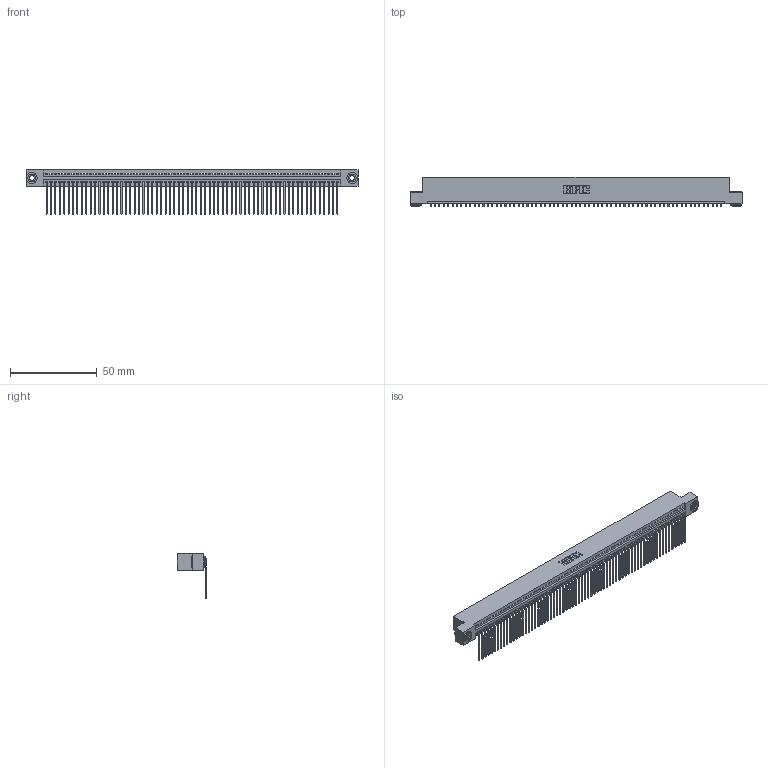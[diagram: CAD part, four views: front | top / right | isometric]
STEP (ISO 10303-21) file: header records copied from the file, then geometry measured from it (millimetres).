
FILE_DESCRIPTION (( 'STEP AP203' ), '1' );
FILE_NAME ('345-067-559-103.STEP', '2018-09-29T05:28:44', ( '' ), ( '' ), 'SwSTEP 2.0', 'SolidWorks 2016', '' );
FILE_SCHEMA (( 'CONFIG_CONTROL_DESIGN' ));
Length unit declared in the file: inch
Products named in the file (4): 345 Part_Flush Mounting Lugs - 0.156 Dia-TH; 345-250-002_345-250-002-102; 345-292-001_558 559 Tail - 1; 345-067-559-103
Assembly tree (70 placements, depth 2):
  345-067-559-103
    345 Part_Flush Mounting Lugs - 0.156 Dia-TH
    345-292-001_558 559 Tail - 1  x67
    345-250-002_345-250-002-102  x2
Bounding box: 191.39 x 16.75 x 25.53 mm (x, y, z)
Volume: 18625.7 mm3; surface area: 26617.9 mm2
Topology: 70 solids, 70 shells, 4184 faces, 12611 edges, 8314 vertices
Faces by surface type: plane 2904, cylinder 1272, cone 8
Entity records: 47794 total; most frequent: CARTESIAN_POINT 8256, ORIENTED_EDGE 8250, DIRECTION 7205, EDGE_CURVE 4125, VECTOR 3701, LINE 3701, VERTEX_POINT 2746, AXIS2_PLACEMENT_3D 1752
